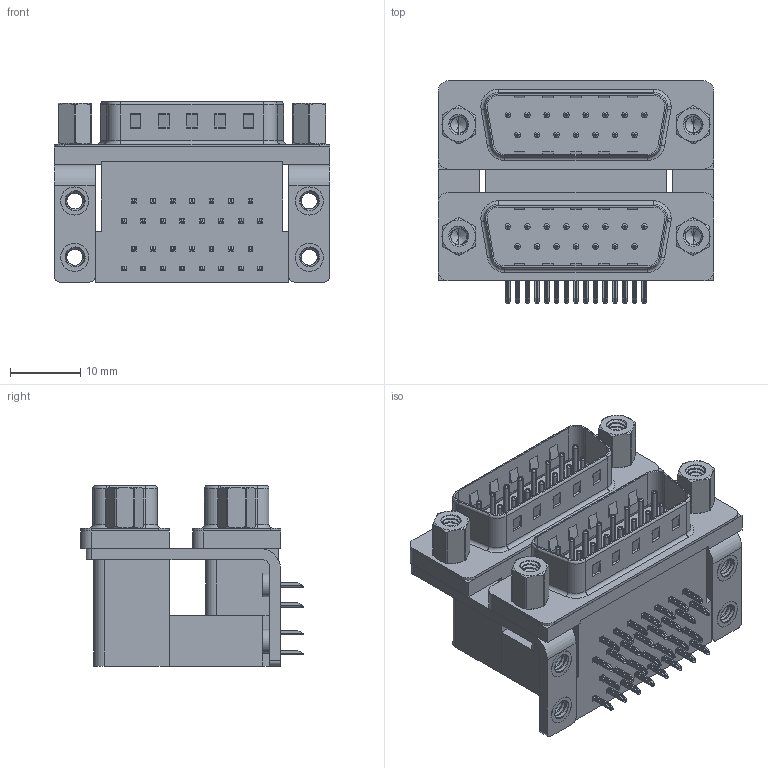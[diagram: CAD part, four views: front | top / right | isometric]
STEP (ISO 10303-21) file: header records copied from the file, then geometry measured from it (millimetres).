
FILE_DESCRIPTION (( 'STEP AP203' ), '1' );
FILE_NAME ('661-015-664-053.STEP', '2022-06-10T23:29:46', ( '' ), ( '' ), 'SwSTEP 2.0', 'SolidWorks 2020', '' );
FILE_SCHEMA (( 'CONFIG_CONTROL_DESIGN' ));
Length unit declared in the file: millimetre
Products named in the file (13): 661-015-664-053; 661 4-40 Threaded Board Mount; 661 Housing Lower_15 Contacts; 661 Housing Spacer_15 Contacts L; 661 Contact Top Upper_L; 661 4-40 Hex Standoff 5; 661 Shell_15 Contacts; 661 Threaded Rivet_4-40; 661 Mounting Bracket_ThruL; 661 Contact Bottom Lower; 661 Housing Upper_15 Contacts L; 661 Contact Top Lower; 661 Contact Bottom Upper_L
Assembly tree (49 placements, depth 2):
  661-015-664-053
    661 Housing Lower_15 Contacts
    661 Housing Spacer_15 Contacts L
    661 Housing Upper_15 Contacts L
    661 Shell_15 Contacts  x2
    661 Contact Bottom Lower  x7
    661 Contact Top Lower  x8
    661 Contact Bottom Upper_L  x7
    661 Contact Top Upper_L  x8
    661 Mounting Bracket_ThruL  x2
    661 4-40 Threaded Board Mount  x4
    661 Threaded Rivet_4-40  x4
    661 4-40 Hex Standoff 5  x4
Bounding box: 39.19 x 31.61 x 25.6 mm (x, y, z)
Volume: 14213.5 mm3; surface area: 16291 mm2
Topology: 49 solids, 49 shells, 3354 faces, 8392 edges, 5226 vertices
Faces by surface type: plane 1890, cylinder 1074, torus 242, cone 100, bspline 48
Entity records: 38518 total; most frequent: CARTESIAN_POINT 11285, DIRECTION 5138, ORIENTED_EDGE 5124, EDGE_CURVE 2562, VECTOR 1752, LINE 1752, AXIS2_PLACEMENT_3D 1693, VERTEX_POINT 1643
